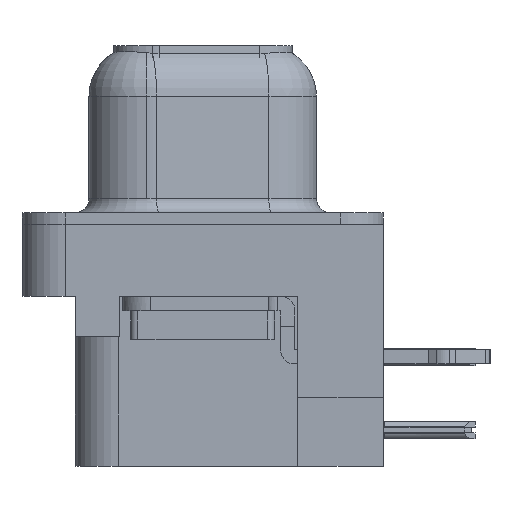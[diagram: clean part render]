
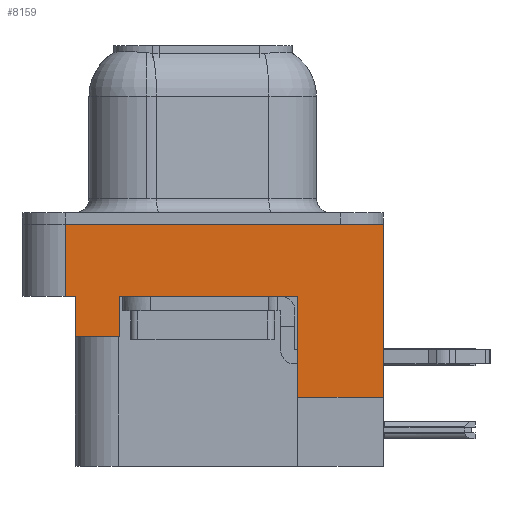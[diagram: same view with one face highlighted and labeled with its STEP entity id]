
A CAD part, left-side view. The second image highlights one B-rep face of the part: STEP entity #8159.
In plain terms, the highlighted planar face has unit normal (-1, 0, 0).
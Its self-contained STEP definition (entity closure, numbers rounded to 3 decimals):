
#171 = CARTESIAN_POINT ( 'NONE',  ( -3., 4.425, -3.9 ) ) ;
#665 = LINE ( 'NONE', #25651, #7053 ) ;
#724 = CARTESIAN_POINT ( 'NONE',  ( -3., 4.425, -3.9 ) ) ;
#1854 = DIRECTION ( 'NONE',  ( 0., 1., 0. ) ) ;
#1992 = DIRECTION ( 'NONE',  ( 0., 0., 1. ) ) ;
#2052 = LINE ( 'NONE', #4417, #12576 ) ;
#2711 = LINE ( 'NONE', #3020, #9101 ) ;
#2939 = DIRECTION ( 'NONE',  ( 0., 0., 1. ) ) ;
#2946 = DIRECTION ( 'NONE',  ( -1., 0., 0. ) ) ;
#2995 = DIRECTION ( 'NONE',  ( 0., 0., 1. ) ) ;
#3020 = CARTESIAN_POINT ( 'NONE',  ( -3., -6.275, -2.5 ) ) ;
#3632 = VERTEX_POINT ( 'NONE', #724 ) ;
#4417 = CARTESIAN_POINT ( 'NONE',  ( -3., -3.295, -8.4 ) ) ;
#4832 = VERTEX_POINT ( 'NONE', #9115 ) ;
#4973 = EDGE_CURVE ( 'NONE', #28314, #7399, #9654, .T. ) ;
#5179 = ORIENTED_EDGE ( 'NONE', *, *, #10983, .F. ) ;
#6189 = ORIENTED_EDGE ( 'NONE', *, *, #15564, .T. ) ;
#6783 = LINE ( 'NONE', #27750, #15404 ) ;
#7053 = VECTOR ( 'NONE', #9016, 1000. ) ;
#7399 = VERTEX_POINT ( 'NONE', #23179 ) ;
#7923 = ORIENTED_EDGE ( 'NONE', *, *, #17746, .F. ) ;
#8159 = ADVANCED_FACE ( 'NONE', ( #24397 ), #29110, .T. ) ;
#8192 = VECTOR ( 'NONE', #2939, 1000. ) ;
#8420 = LINE ( 'NONE', #19689, #14784 ) ;
#9016 = DIRECTION ( 'NONE',  ( 0., 0., 1. ) ) ;
#9101 = VECTOR ( 'NONE', #10276, 1000. ) ;
#9115 = CARTESIAN_POINT ( 'NONE',  ( -3., 4.775, -2.5 ) ) ;
#9654 = LINE ( 'NONE', #25225, #21528 ) ;
#9738 = EDGE_CURVE ( 'NONE', #4832, #21984, #2711, .T. ) ;
#9823 = CARTESIAN_POINT ( 'NONE',  ( -3., -6.275, -6. ) ) ;
#10087 = VERTEX_POINT ( 'NONE', #28140 ) ;
#10276 = DIRECTION ( 'NONE',  ( 0., -1., 0. ) ) ;
#10679 = ORIENTED_EDGE ( 'NONE', *, *, #9738, .T. ) ;
#10782 = DIRECTION ( 'NONE',  ( 0., -1., 0. ) ) ;
#10983 = EDGE_CURVE ( 'NONE', #23581, #3632, #6783, .T. ) ;
#11326 = CARTESIAN_POINT ( 'NONE',  ( -3., -6.495, -6. ) ) ;
#11437 = EDGE_CURVE ( 'NONE', #22575, #27691, #27241, .T. ) ;
#11680 = CARTESIAN_POINT ( 'NONE',  ( -3., 4.425, -2.5 ) ) ;
#11833 = LINE ( 'NONE', #24963, #30771 ) ;
#12163 = EDGE_CURVE ( 'NONE', #4832, #28314, #26434, .T. ) ;
#12407 = AXIS2_PLACEMENT_3D ( 'NONE', #17282, #2946, #19649 ) ;
#12469 = EDGE_CURVE ( 'NONE', #22575, #7399, #665, .T. ) ;
#12576 = VECTOR ( 'NONE', #1992, 1000. ) ;
#12595 = CARTESIAN_POINT ( 'NONE',  ( -3., -3.295, -6. ) ) ;
#13779 = EDGE_LOOP ( 'NONE', ( #29504, #24185, #23033, #22546, #10679, #7923, #5179, #20940, #6189, #16561 ) ) ;
#14616 = VECTOR ( 'NONE', #1854, 1000. ) ;
#14784 = VECTOR ( 'NONE', #2995, 1000. ) ;
#15404 = VECTOR ( 'NONE', #25450, 1000. ) ;
#15429 = EDGE_CURVE ( 'NONE', #23581, #17904, #8420, .T. ) ;
#15564 = EDGE_CURVE ( 'NONE', #17904, #10087, #11833, .T. ) ;
#16169 = LINE ( 'NONE', #171, #29547 ) ;
#16561 = ORIENTED_EDGE ( 'NONE', *, *, #30714, .F. ) ;
#16917 = DIRECTION ( 'NONE',  ( 0., 0., 1. ) ) ;
#17282 = CARTESIAN_POINT ( 'NONE',  ( -3., -6.275, -2.5 ) ) ;
#17744 = CARTESIAN_POINT ( 'NONE',  ( -3., 2.895, -2.5 ) ) ;
#17746 = EDGE_CURVE ( 'NONE', #3632, #21984, #16169, .T. ) ;
#17904 = VERTEX_POINT ( 'NONE', #17744 ) ;
#19644 = CARTESIAN_POINT ( 'NONE',  ( -3., 4.775, -2.5 ) ) ;
#19649 = DIRECTION ( 'NONE',  ( 0., 0., 1. ) ) ;
#19689 = CARTESIAN_POINT ( 'NONE',  ( -3., 2.895, -3.9 ) ) ;
#20940 = ORIENTED_EDGE ( 'NONE', *, *, #15429, .T. ) ;
#20983 = CARTESIAN_POINT ( 'NONE',  ( -3., 2.895, -3.9 ) ) ;
#21528 = VECTOR ( 'NONE', #22481, 1000. ) ;
#21984 = VERTEX_POINT ( 'NONE', #11680 ) ;
#22481 = DIRECTION ( 'NONE',  ( 0., -1., 0. ) ) ;
#22546 = ORIENTED_EDGE ( 'NONE', *, *, #12163, .F. ) ;
#22575 = VERTEX_POINT ( 'NONE', #9823 ) ;
#23033 = ORIENTED_EDGE ( 'NONE', *, *, #4973, .F. ) ;
#23179 = CARTESIAN_POINT ( 'NONE',  ( -3., -6.275, 0. ) ) ;
#23581 = VERTEX_POINT ( 'NONE', #20983 ) ;
#24185 = ORIENTED_EDGE ( 'NONE', *, *, #12469, .T. ) ;
#24333 = CARTESIAN_POINT ( 'NONE',  ( -3., 4.775, 0. ) ) ;
#24397 = FACE_OUTER_BOUND ( 'NONE', #13779, .T. ) ;
#24963 = CARTESIAN_POINT ( 'NONE',  ( -3., -6.275, -2.5 ) ) ;
#25225 = CARTESIAN_POINT ( 'NONE',  ( -3., -6.275, 0. ) ) ;
#25450 = DIRECTION ( 'NONE',  ( 0., 1., 0. ) ) ;
#25651 = CARTESIAN_POINT ( 'NONE',  ( -3., -6.275, -2.5 ) ) ;
#26434 = LINE ( 'NONE', #19644, #8192 ) ;
#27241 = LINE ( 'NONE', #11326, #14616 ) ;
#27691 = VERTEX_POINT ( 'NONE', #12595 ) ;
#27750 = CARTESIAN_POINT ( 'NONE',  ( -3., 4.425, -3.9 ) ) ;
#28140 = CARTESIAN_POINT ( 'NONE',  ( -3., -3.295, -2.5 ) ) ;
#28314 = VERTEX_POINT ( 'NONE', #24333 ) ;
#29110 = PLANE ( 'NONE',  #12407 ) ;
#29504 = ORIENTED_EDGE ( 'NONE', *, *, #11437, .F. ) ;
#29547 = VECTOR ( 'NONE', #16917, 1000. ) ;
#30714 = EDGE_CURVE ( 'NONE', #27691, #10087, #2052, .T. ) ;
#30771 = VECTOR ( 'NONE', #10782, 1000. ) ;
